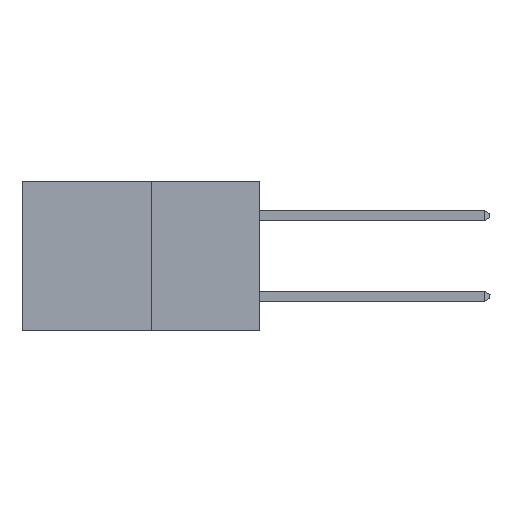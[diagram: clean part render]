
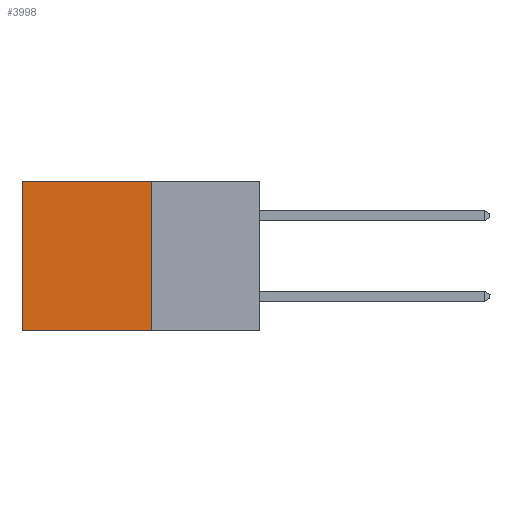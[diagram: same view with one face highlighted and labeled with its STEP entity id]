
A CAD part, left-side view. The second image highlights one B-rep face of the part: STEP entity #3998.
In plain terms, the highlighted planar face has unit normal (-1, 0, 0).
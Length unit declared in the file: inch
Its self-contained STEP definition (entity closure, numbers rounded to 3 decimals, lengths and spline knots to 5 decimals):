
#140 = CARTESIAN_POINT ( 'NONE',  ( 0.277, 0.59, 0. ) ) ;
#369 = EDGE_CURVE ( 'NONE', #6498, #9329, #6682, .T. ) ;
#461 = VERTEX_POINT ( 'NONE', #4235 ) ;
#668 = CARTESIAN_POINT ( 'NONE',  ( 0.277, 0.27, 0. ) ) ;
#950 = VECTOR ( 'NONE', #7028, 39.37008 ) ;
#1252 = LINE ( 'NONE', #2569, #950 ) ;
#1459 = DIRECTION ( 'NONE',  ( 0., 1., 0. ) ) ;
#1577 = EDGE_CURVE ( 'NONE', #8751, #6498, #3472, .T. ) ;
#1644 = LINE ( 'NONE', #5411, #9249 ) ;
#1876 = CARTESIAN_POINT ( 'NONE',  ( 0.277, 0.27, 0. ) ) ;
#2080 = EDGE_CURVE ( 'NONE', #461, #9329, #1644, .T. ) ;
#2340 = ORIENTED_EDGE ( 'NONE', *, *, #369, .T. ) ;
#2569 = CARTESIAN_POINT ( 'NONE',  ( 0.277, 0.27, -0.37 ) ) ;
#2820 = VECTOR ( 'NONE', #8170, 39.37008 ) ;
#3472 = LINE ( 'NONE', #1876, #7109 ) ;
#3998 = ADVANCED_FACE ( 'NONE', ( #9670 ), #4489, .F. ) ;
#4235 = CARTESIAN_POINT ( 'NONE',  ( 0.277, 0.27, -0.37 ) ) ;
#4489 = PLANE ( 'NONE',  #5985 ) ;
#4607 = DIRECTION ( 'NONE',  ( 0., 0., -1. ) ) ;
#4885 = DIRECTION ( 'NONE',  ( 1., 0., 0. ) ) ;
#5411 = CARTESIAN_POINT ( 'NONE',  ( 0.277, 0.27, -0.37 ) ) ;
#5985 = AXIS2_PLACEMENT_3D ( 'NONE', #6420, #4885, #4607 ) ;
#6070 = ORIENTED_EDGE ( 'NONE', *, *, #8304, .F. ) ;
#6103 = ORIENTED_EDGE ( 'NONE', *, *, #1577, .T. ) ;
#6206 = DIRECTION ( 'NONE',  ( 0., 1., 0. ) ) ;
#6420 = CARTESIAN_POINT ( 'NONE',  ( 0.277, 0.27, -0.37 ) ) ;
#6498 = VERTEX_POINT ( 'NONE', #140 ) ;
#6682 = LINE ( 'NONE', #8317, #2820 ) ;
#7028 = DIRECTION ( 'NONE',  ( 0., 0., -1. ) ) ;
#7109 = VECTOR ( 'NONE', #6206, 39.37008 ) ;
#7697 = EDGE_LOOP ( 'NONE', ( #2340, #9052, #6070, #6103 ) ) ;
#8170 = DIRECTION ( 'NONE',  ( 0., 0., -1. ) ) ;
#8304 = EDGE_CURVE ( 'NONE', #8751, #461, #1252, .T. ) ;
#8317 = CARTESIAN_POINT ( 'NONE',  ( 0.277, 0.59, -0.37 ) ) ;
#8408 = CARTESIAN_POINT ( 'NONE',  ( 0.277, 0.59, -0.37 ) ) ;
#8751 = VERTEX_POINT ( 'NONE', #668 ) ;
#9052 = ORIENTED_EDGE ( 'NONE', *, *, #2080, .F. ) ;
#9249 = VECTOR ( 'NONE', #1459, 39.37008 ) ;
#9329 = VERTEX_POINT ( 'NONE', #8408 ) ;
#9670 = FACE_OUTER_BOUND ( 'NONE', #7697, .T. ) ;
